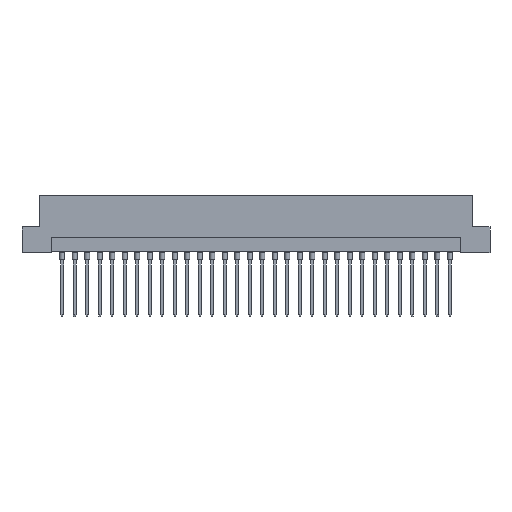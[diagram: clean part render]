
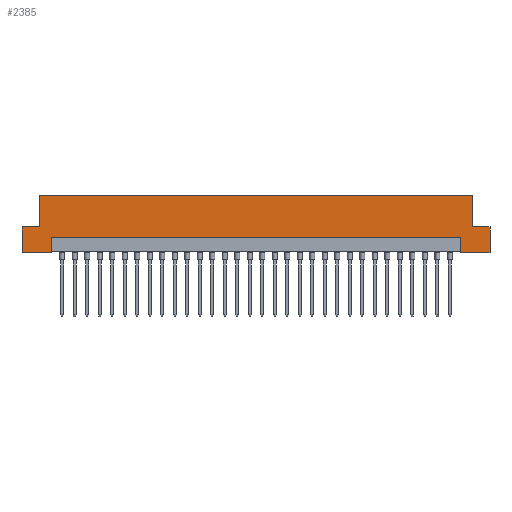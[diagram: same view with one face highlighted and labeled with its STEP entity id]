
A CAD part, front view. The second image highlights one B-rep face of the part: STEP entity #2385.
In plain terms, the highlighted planar face has unit normal (0, -1, 0).
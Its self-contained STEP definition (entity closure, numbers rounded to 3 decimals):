
#94 = DIRECTION ( 'NONE',  ( 0., 0., 1. ) ) ;
#141 = EDGE_CURVE ( 'NONE', #9383, #4660, #7499, .T. ) ;
#199 = CARTESIAN_POINT ( 'NONE',  ( -47.5, -4.3, 0. ) ) ;
#413 = VECTOR ( 'NONE', #8291, 1000. ) ;
#570 = DIRECTION ( 'NONE',  ( 1., 0., 0. ) ) ;
#613 = EDGE_CURVE ( 'NONE', #10810, #4660, #4483, .T. ) ;
#876 = CARTESIAN_POINT ( 'NONE',  ( -41.6, -4.3, 3. ) ) ;
#985 = VERTEX_POINT ( 'NONE', #12036 ) ;
#986 = VERTEX_POINT ( 'NONE', #2575 ) ;
#1299 = CARTESIAN_POINT ( 'NONE',  ( 47.5, -4.3, 5.2 ) ) ;
#1304 = CARTESIAN_POINT ( 'NONE',  ( 47.5, -4.3, 0. ) ) ;
#1357 = EDGE_CURVE ( 'NONE', #986, #3377, #5608, .T. ) ;
#1394 = ORIENTED_EDGE ( 'NONE', *, *, #8529, .F. ) ;
#1716 = DIRECTION ( 'NONE',  ( 0., 1., 0. ) ) ;
#1928 = VERTEX_POINT ( 'NONE', #3807 ) ;
#1933 = CARTESIAN_POINT ( 'NONE',  ( 44., -4.3, 11.6 ) ) ;
#2007 = EDGE_CURVE ( 'NONE', #1928, #3377, #9724, .T. ) ;
#2064 = VERTEX_POINT ( 'NONE', #5773 ) ;
#2132 = EDGE_CURVE ( 'NONE', #986, #7965, #9667, .T. ) ;
#2276 = CARTESIAN_POINT ( 'NONE',  ( 41.6, -4.3, 3. ) ) ;
#2385 = ADVANCED_FACE ( 'NONE', ( #4468 ), #7414, .F. ) ;
#2534 = VECTOR ( 'NONE', #5035, 1000. ) ;
#2575 = CARTESIAN_POINT ( 'NONE',  ( 44., -4.3, 5.2 ) ) ;
#2657 = CARTESIAN_POINT ( 'NONE',  ( -41.6, -4.3, 3. ) ) ;
#2841 = CARTESIAN_POINT ( 'NONE',  ( -41.6, -4.3, 0.2 ) ) ;
#3007 = DIRECTION ( 'NONE',  ( 1., 0., 0. ) ) ;
#3097 = VECTOR ( 'NONE', #7247, 1000. ) ;
#3228 = VECTOR ( 'NONE', #3007, 1000. ) ;
#3289 = ORIENTED_EDGE ( 'NONE', *, *, #7270, .F. ) ;
#3318 = CARTESIAN_POINT ( 'NONE',  ( -44., -4.3, 5.2 ) ) ;
#3377 = VERTEX_POINT ( 'NONE', #1933 ) ;
#3478 = DIRECTION ( 'NONE',  ( 1., 0., 0. ) ) ;
#3575 = ORIENTED_EDGE ( 'NONE', *, *, #5588, .F. ) ;
#3654 = VERTEX_POINT ( 'NONE', #5198 ) ;
#3737 = CARTESIAN_POINT ( 'NONE',  ( 41.6, -4.3, 0.2 ) ) ;
#3807 = CARTESIAN_POINT ( 'NONE',  ( -44., -4.3, 11.6 ) ) ;
#4395 = LINE ( 'NONE', #8135, #6538 ) ;
#4468 = FACE_OUTER_BOUND ( 'NONE', #5120, .T. ) ;
#4483 = LINE ( 'NONE', #11254, #6295 ) ;
#4609 = DIRECTION ( 'NONE',  ( 1., 0., 0. ) ) ;
#4660 = VERTEX_POINT ( 'NONE', #5689 ) ;
#4749 = VECTOR ( 'NONE', #570, 1000. ) ;
#4990 = VECTOR ( 'NONE', #7850, 1000. ) ;
#5035 = DIRECTION ( 'NONE',  ( 0., 0., 1. ) ) ;
#5120 = EDGE_LOOP ( 'NONE', ( #11719, #3289, #8505, #6331, #5602, #11846, #6031, #3575, #1394, #11086, #11944, #9469 ) ) ;
#5198 = CARTESIAN_POINT ( 'NONE',  ( 47.5, -4.3, 0. ) ) ;
#5390 = EDGE_CURVE ( 'NONE', #7965, #3654, #9016, .T. ) ;
#5588 = EDGE_CURVE ( 'NONE', #985, #1928, #7979, .T. ) ;
#5602 = ORIENTED_EDGE ( 'NONE', *, *, #2132, .F. ) ;
#5608 = LINE ( 'NONE', #7625, #7334 ) ;
#5689 = CARTESIAN_POINT ( 'NONE',  ( -41.6, -4.3, 0. ) ) ;
#5773 = CARTESIAN_POINT ( 'NONE',  ( -47.5, -4.3, 5.2 ) ) ;
#6031 = ORIENTED_EDGE ( 'NONE', *, *, #2007, .F. ) ;
#6106 = VERTEX_POINT ( 'NONE', #11653 ) ;
#6271 = EDGE_CURVE ( 'NONE', #2064, #10810, #9273, .T. ) ;
#6295 = VECTOR ( 'NONE', #6564, 1000. ) ;
#6310 = VECTOR ( 'NONE', #10278, 1000. ) ;
#6331 = ORIENTED_EDGE ( 'NONE', *, *, #5390, .F. ) ;
#6538 = VECTOR ( 'NONE', #3478, 1000. ) ;
#6564 = DIRECTION ( 'NONE',  ( 1., 0., 0. ) ) ;
#6676 = LINE ( 'NONE', #3737, #6310 ) ;
#7035 = EDGE_CURVE ( 'NONE', #6106, #3654, #10766, .T. ) ;
#7247 = DIRECTION ( 'NONE',  ( 0., 0., -1. ) ) ;
#7270 = EDGE_CURVE ( 'NONE', #6106, #11285, #6676, .T. ) ;
#7334 = VECTOR ( 'NONE', #94, 1000. ) ;
#7414 = PLANE ( 'NONE',  #7415 ) ;
#7415 = AXIS2_PLACEMENT_3D ( 'NONE', #9229, #1716, #10272 ) ;
#7499 = LINE ( 'NONE', #2841, #413 ) ;
#7625 = CARTESIAN_POINT ( 'NONE',  ( 44., -4.3, 5.2 ) ) ;
#7850 = DIRECTION ( 'NONE',  ( 1., 0., 0. ) ) ;
#7965 = VERTEX_POINT ( 'NONE', #10606 ) ;
#7979 = LINE ( 'NONE', #3318, #2534 ) ;
#8135 = CARTESIAN_POINT ( 'NONE',  ( -47.5, -4.3, 5.2 ) ) ;
#8291 = DIRECTION ( 'NONE',  ( 0., 0., -1. ) ) ;
#8402 = VECTOR ( 'NONE', #10247, 1000. ) ;
#8505 = ORIENTED_EDGE ( 'NONE', *, *, #7035, .T. ) ;
#8529 = EDGE_CURVE ( 'NONE', #2064, #985, #4395, .T. ) ;
#9016 = LINE ( 'NONE', #9250, #3097 ) ;
#9229 = CARTESIAN_POINT ( 'NONE',  ( 47.5, -4.3, 11.6 ) ) ;
#9250 = CARTESIAN_POINT ( 'NONE',  ( 47.5, -4.3, 11.6 ) ) ;
#9251 = LINE ( 'NONE', #2657, #9865 ) ;
#9273 = LINE ( 'NONE', #11099, #8402 ) ;
#9383 = VERTEX_POINT ( 'NONE', #876 ) ;
#9469 = ORIENTED_EDGE ( 'NONE', *, *, #141, .F. ) ;
#9491 = CARTESIAN_POINT ( 'NONE',  ( 47.5, -4.3, 11.6 ) ) ;
#9667 = LINE ( 'NONE', #1299, #4990 ) ;
#9724 = LINE ( 'NONE', #9491, #3228 ) ;
#9865 = VECTOR ( 'NONE', #4609, 1000. ) ;
#10247 = DIRECTION ( 'NONE',  ( 0., 0., -1. ) ) ;
#10272 = DIRECTION ( 'NONE',  ( -1., 0., 0. ) ) ;
#10278 = DIRECTION ( 'NONE',  ( 0., 0., 1. ) ) ;
#10606 = CARTESIAN_POINT ( 'NONE',  ( 47.5, -4.3, 5.2 ) ) ;
#10766 = LINE ( 'NONE', #1304, #4749 ) ;
#10810 = VERTEX_POINT ( 'NONE', #199 ) ;
#11086 = ORIENTED_EDGE ( 'NONE', *, *, #6271, .T. ) ;
#11099 = CARTESIAN_POINT ( 'NONE',  ( -47.5, -4.3, 11.6 ) ) ;
#11254 = CARTESIAN_POINT ( 'NONE',  ( 47.5, -4.3, 0. ) ) ;
#11285 = VERTEX_POINT ( 'NONE', #2276 ) ;
#11653 = CARTESIAN_POINT ( 'NONE',  ( 41.6, -4.3, 0. ) ) ;
#11719 = ORIENTED_EDGE ( 'NONE', *, *, #12017, .T. ) ;
#11846 = ORIENTED_EDGE ( 'NONE', *, *, #1357, .T. ) ;
#11944 = ORIENTED_EDGE ( 'NONE', *, *, #613, .T. ) ;
#12017 = EDGE_CURVE ( 'NONE', #9383, #11285, #9251, .T. ) ;
#12036 = CARTESIAN_POINT ( 'NONE',  ( -44., -4.3, 5.2 ) ) ;
